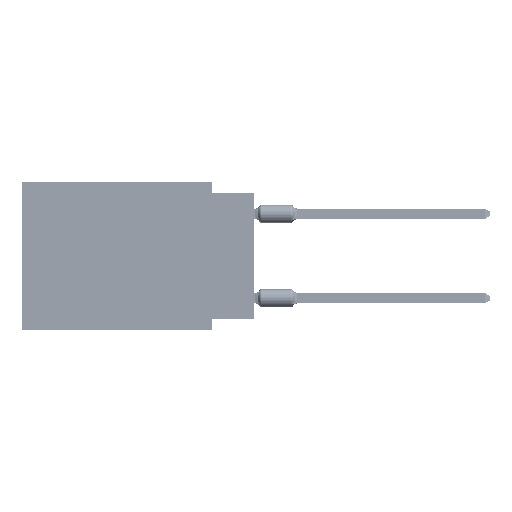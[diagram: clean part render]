
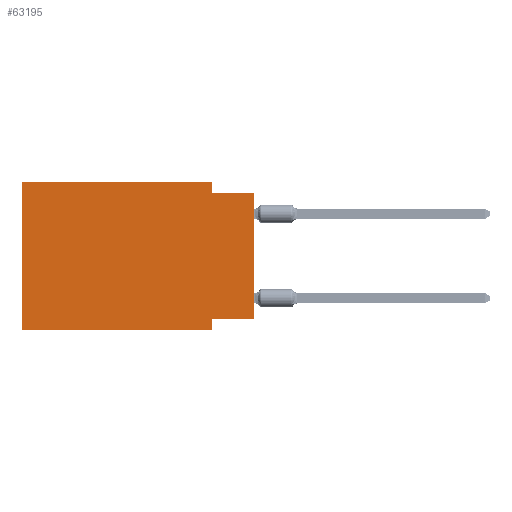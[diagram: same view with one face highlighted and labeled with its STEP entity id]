
A CAD part, left-side view. The second image highlights one B-rep face of the part: STEP entity #63195.
In plain terms, the highlighted planar face has unit normal (-1, 0, 0).
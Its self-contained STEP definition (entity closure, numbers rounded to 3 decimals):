
#1113 = CARTESIAN_POINT ( 'NONE',  ( 0., 13.97, -8.89 ) ) ;
#2007 = VECTOR ( 'NONE', #15530, 1000. ) ;
#2047 = DIRECTION ( 'NONE',  ( 0., 0., -1. ) ) ;
#5515 = VERTEX_POINT ( 'NONE', #1113 ) ;
#5948 = VECTOR ( 'NONE', #22540, 1000. ) ;
#6738 = LINE ( 'NONE', #20078, #39616 ) ;
#7008 = ORIENTED_EDGE ( 'NONE', *, *, #19705, .T. ) ;
#7027 = VERTEX_POINT ( 'NONE', #46867 ) ;
#7354 = FACE_OUTER_BOUND ( 'NONE', #52860, .T. ) ;
#8123 = EDGE_CURVE ( 'NONE', #46844, #30243, #61827, .T. ) ;
#9504 = ORIENTED_EDGE ( 'NONE', *, *, #52116, .F. ) ;
#10177 = LINE ( 'NONE', #44428, #2007 ) ;
#11439 = VERTEX_POINT ( 'NONE', #32660 ) ;
#12112 = VERTEX_POINT ( 'NONE', #75232 ) ;
#13236 = VECTOR ( 'NONE', #68557, 1000. ) ;
#14566 = DIRECTION ( 'NONE',  ( 0., 0., 1. ) ) ;
#15450 = LINE ( 'NONE', #44351, #18128 ) ;
#15463 = VERTEX_POINT ( 'NONE', #47993 ) ;
#15530 = DIRECTION ( 'NONE',  ( 0., 0., 1. ) ) ;
#18128 = VECTOR ( 'NONE', #38664, 1000. ) ;
#18221 = ORIENTED_EDGE ( 'NONE', *, *, #8123, .F. ) ;
#19705 = EDGE_CURVE ( 'NONE', #7027, #11439, #10177, .T. ) ;
#20078 = CARTESIAN_POINT ( 'NONE',  ( 0., 2.54, -8.89 ) ) ;
#20786 = ORIENTED_EDGE ( 'NONE', *, *, #59816, .F. ) ;
#21396 = EDGE_CURVE ( 'NONE', #7027, #15463, #15450, .T. ) ;
#21831 = CARTESIAN_POINT ( 'NONE',  ( 0., 13.97, 0. ) ) ;
#22540 = DIRECTION ( 'NONE',  ( 0., -1., 0. ) ) ;
#22562 = DIRECTION ( 'NONE',  ( 0., -1., 0. ) ) ;
#24832 = CARTESIAN_POINT ( 'NONE',  ( 0., 13.97, 0. ) ) ;
#27491 = LINE ( 'NONE', #51117, #5948 ) ;
#28575 = CARTESIAN_POINT ( 'NONE',  ( 0., 2.54, -0.635 ) ) ;
#29310 = ORIENTED_EDGE ( 'NONE', *, *, #66010, .F. ) ;
#30243 = VERTEX_POINT ( 'NONE', #28575 ) ;
#30691 = ORIENTED_EDGE ( 'NONE', *, *, #50006, .F. ) ;
#32660 = CARTESIAN_POINT ( 'NONE',  ( 0., 0., -0.635 ) ) ;
#35039 = CARTESIAN_POINT ( 'NONE',  ( 0., 2.54, 0. ) ) ;
#36812 = DIRECTION ( 'NONE',  ( 0., 0., -1. ) ) ;
#38298 = ORIENTED_EDGE ( 'NONE', *, *, #60191, .T. ) ;
#38664 = DIRECTION ( 'NONE',  ( 0., 1., 0. ) ) ;
#39616 = VECTOR ( 'NONE', #36812, 1000. ) ;
#43480 = CARTESIAN_POINT ( 'NONE',  ( 0., 13.97, 0. ) ) ;
#43529 = VERTEX_POINT ( 'NONE', #24832 ) ;
#44351 = CARTESIAN_POINT ( 'NONE',  ( 0., 0., -8.255 ) ) ;
#44428 = CARTESIAN_POINT ( 'NONE',  ( 0., 0., 0. ) ) ;
#45263 = CARTESIAN_POINT ( 'NONE',  ( 0., 13.97, -8.89 ) ) ;
#45391 = VECTOR ( 'NONE', #22562, 1000. ) ;
#46572 = PLANE ( 'NONE',  #62080 ) ;
#46844 = VERTEX_POINT ( 'NONE', #35039 ) ;
#46867 = CARTESIAN_POINT ( 'NONE',  ( 0., 0., -8.255 ) ) ;
#47993 = CARTESIAN_POINT ( 'NONE',  ( 0., 2.54, -8.255 ) ) ;
#48075 = DIRECTION ( 'NONE',  ( 1., 0., 0. ) ) ;
#49209 = LINE ( 'NONE', #43480, #52524 ) ;
#49737 = LINE ( 'NONE', #21831, #45391 ) ;
#50006 = EDGE_CURVE ( 'NONE', #15463, #12112, #6738, .T. ) ;
#51117 = CARTESIAN_POINT ( 'NONE',  ( 0., 0., -0.635 ) ) ;
#52116 = EDGE_CURVE ( 'NONE', #5515, #43529, #49209, .T. ) ;
#52524 = VECTOR ( 'NONE', #14566, 1000. ) ;
#52860 = EDGE_LOOP ( 'NONE', ( #7008, #20786, #18221, #29310, #9504, #38298, #30691, #58615 ) ) ;
#53814 = CARTESIAN_POINT ( 'NONE',  ( 0., 13.97, 0. ) ) ;
#54220 = CARTESIAN_POINT ( 'NONE',  ( 0., 2.54, 0. ) ) ;
#57871 = LINE ( 'NONE', #45263, #13236 ) ;
#58615 = ORIENTED_EDGE ( 'NONE', *, *, #21396, .F. ) ;
#59816 = EDGE_CURVE ( 'NONE', #30243, #11439, #27491, .T. ) ;
#60191 = EDGE_CURVE ( 'NONE', #5515, #12112, #57871, .T. ) ;
#61827 = LINE ( 'NONE', #54220, #68500 ) ;
#62080 = AXIS2_PLACEMENT_3D ( 'NONE', #53814, #48075, #71365 ) ;
#63195 = ADVANCED_FACE ( 'NONE', ( #7354 ), #46572, .F. ) ;
#66010 = EDGE_CURVE ( 'NONE', #43529, #46844, #49737, .T. ) ;
#68500 = VECTOR ( 'NONE', #2047, 1000. ) ;
#68557 = DIRECTION ( 'NONE',  ( 0., -1., 0. ) ) ;
#71365 = DIRECTION ( 'NONE',  ( 0., 0., -1. ) ) ;
#75232 = CARTESIAN_POINT ( 'NONE',  ( 0., 2.54, -8.89 ) ) ;
